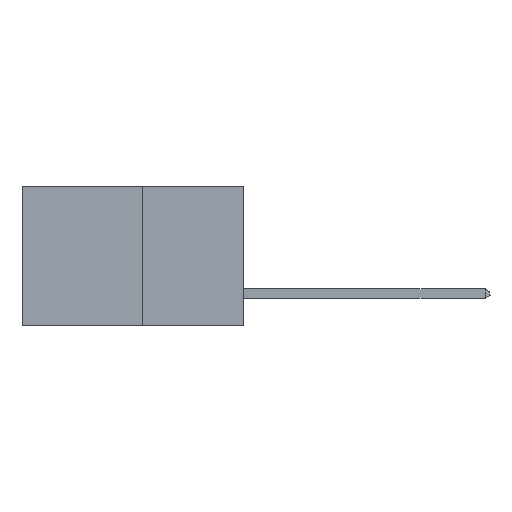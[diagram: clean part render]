
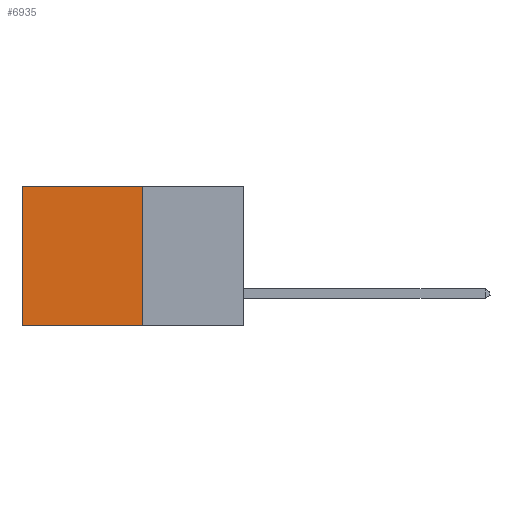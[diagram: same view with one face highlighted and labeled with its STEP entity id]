
A CAD part, left-side view. The second image highlights one B-rep face of the part: STEP entity #6935.
In plain terms, the highlighted planar face has unit normal (-1, 0, 0).
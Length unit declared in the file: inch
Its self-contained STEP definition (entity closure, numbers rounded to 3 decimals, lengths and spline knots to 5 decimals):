
#243 = CARTESIAN_POINT ( 'NONE',  ( 0.277, 0.59, -0.37 ) ) ;
#613 = LINE ( 'NONE', #8614, #5957 ) ;
#948 = EDGE_CURVE ( 'NONE', #9174, #8094, #613, .T. ) ;
#1293 = EDGE_CURVE ( 'NONE', #9014, #8094, #2554, .T. ) ;
#1948 = EDGE_CURVE ( 'NONE', #10700, #9174, #13062, .T. ) ;
#2263 = ORIENTED_EDGE ( 'NONE', *, *, #1948, .F. ) ;
#2464 = VECTOR ( 'NONE', #9319, 39.37008 ) ;
#2554 = LINE ( 'NONE', #6809, #5169 ) ;
#2984 = FACE_OUTER_BOUND ( 'NONE', #7139, .T. ) ;
#3538 = CARTESIAN_POINT ( 'NONE',  ( 0.277, 0.27, -0.37 ) ) ;
#3846 = ORIENTED_EDGE ( 'NONE', *, *, #1293, .T. ) ;
#4662 = DIRECTION ( 'NONE',  ( 0., 0., -1. ) ) ;
#5036 = CARTESIAN_POINT ( 'NONE',  ( 0.277, 0.27, -0.37 ) ) ;
#5169 = VECTOR ( 'NONE', #12694, 39.37008 ) ;
#5203 = EDGE_CURVE ( 'NONE', #10700, #9014, #6663, .T. ) ;
#5957 = VECTOR ( 'NONE', #9423, 39.37008 ) ;
#6663 = LINE ( 'NONE', #13120, #8952 ) ;
#6809 = CARTESIAN_POINT ( 'NONE',  ( 0.277, 0.59, -0.37 ) ) ;
#6935 = ADVANCED_FACE ( 'NONE', ( #2984 ), #9532, .F. ) ;
#7058 = ORIENTED_EDGE ( 'NONE', *, *, #948, .F. ) ;
#7139 = EDGE_LOOP ( 'NONE', ( #3846, #7058, #2263, #8414 ) ) ;
#7784 = CARTESIAN_POINT ( 'NONE',  ( 0.277, 0.59, 0. ) ) ;
#8094 = VERTEX_POINT ( 'NONE', #243 ) ;
#8414 = ORIENTED_EDGE ( 'NONE', *, *, #5203, .T. ) ;
#8614 = CARTESIAN_POINT ( 'NONE',  ( 0.277, 0.27, -0.37 ) ) ;
#8952 = VECTOR ( 'NONE', #9409, 39.37008 ) ;
#9014 = VERTEX_POINT ( 'NONE', #7784 ) ;
#9147 = AXIS2_PLACEMENT_3D ( 'NONE', #3538, #10486, #4662 ) ;
#9174 = VERTEX_POINT ( 'NONE', #5036 ) ;
#9319 = DIRECTION ( 'NONE',  ( 0., 0., -1. ) ) ;
#9409 = DIRECTION ( 'NONE',  ( 0., 1., 0. ) ) ;
#9423 = DIRECTION ( 'NONE',  ( 0., 1., 0. ) ) ;
#9516 = CARTESIAN_POINT ( 'NONE',  ( 0.277, 0.27, 0. ) ) ;
#9532 = PLANE ( 'NONE',  #9147 ) ;
#10486 = DIRECTION ( 'NONE',  ( 1., 0., 0. ) ) ;
#10700 = VERTEX_POINT ( 'NONE', #9516 ) ;
#12094 = CARTESIAN_POINT ( 'NONE',  ( 0.277, 0.27, -0.37 ) ) ;
#12694 = DIRECTION ( 'NONE',  ( 0., 0., -1. ) ) ;
#13062 = LINE ( 'NONE', #12094, #2464 ) ;
#13120 = CARTESIAN_POINT ( 'NONE',  ( 0.277, 0.27, 0. ) ) ;
